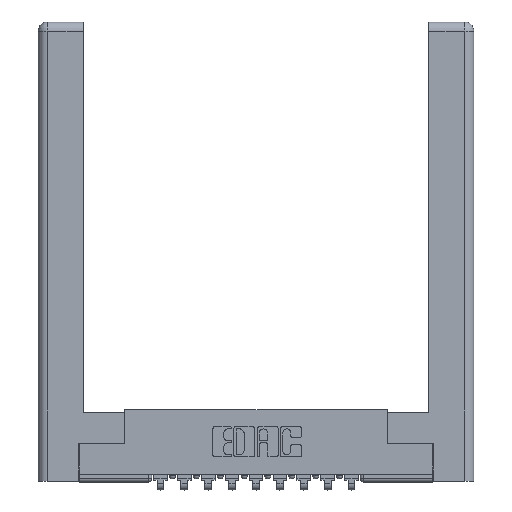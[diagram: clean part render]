
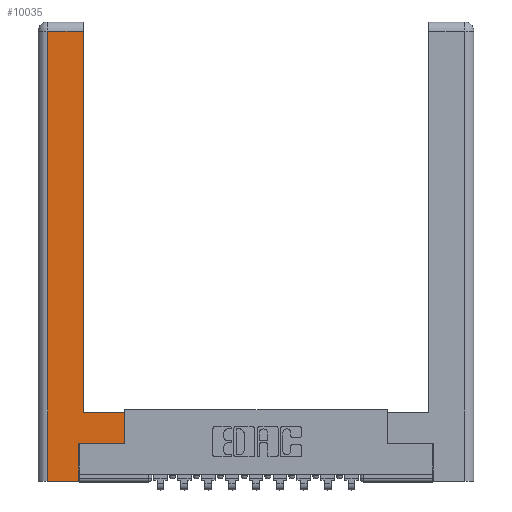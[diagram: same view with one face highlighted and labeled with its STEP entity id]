
A CAD part, top view. The second image highlights one B-rep face of the part: STEP entity #10035.
In plain terms, the highlighted planar face has unit normal (0, 0, 1).
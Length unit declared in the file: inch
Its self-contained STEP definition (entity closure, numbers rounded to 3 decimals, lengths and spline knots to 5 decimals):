
#168 = DIRECTION ( 'NONE',  ( 0., -1., 0. ) ) ;
#281 = CARTESIAN_POINT ( 'NONE',  ( 0., 0., 0. ) ) ;
#720 = ORIENTED_EDGE ( 'NONE', *, *, #9468, .T. ) ;
#917 = AXIS2_PLACEMENT_3D ( 'NONE', #281, #7357, #5945 ) ;
#1008 = LINE ( 'NONE', #1153, #5351 ) ;
#1153 = CARTESIAN_POINT ( 'NONE',  ( 0.265, 0., 0. ) ) ;
#1521 = EDGE_CURVE ( 'NONE', #10462, #13008, #4277, .T. ) ;
#1778 = CARTESIAN_POINT ( 'NONE',  ( 0.0615, 2.94, 0. ) ) ;
#1956 = VECTOR ( 'NONE', #4192, 39.37008 ) ;
#1999 = CARTESIAN_POINT ( 'NONE',  ( 0.565, 0.245, 0. ) ) ;
#2003 = FACE_OUTER_BOUND ( 'NONE', #11469, .T. ) ;
#2442 = EDGE_CURVE ( 'NONE', #12706, #10462, #7905, .T. ) ;
#2484 = LINE ( 'NONE', #15173, #7563 ) ;
#2895 = VERTEX_POINT ( 'NONE', #4299 ) ;
#2990 = DIRECTION ( 'NONE',  ( 0., 1., 0. ) ) ;
#4166 = EDGE_CURVE ( 'NONE', #12667, #4741, #8898, .T. ) ;
#4192 = DIRECTION ( 'NONE',  ( 0., 1., 0. ) ) ;
#4277 = LINE ( 'NONE', #9017, #11443 ) ;
#4299 = CARTESIAN_POINT ( 'NONE',  ( 0.0615, 0., 0. ) ) ;
#4522 = DIRECTION ( 'NONE',  ( -1., 0., 0. ) ) ;
#4537 = CARTESIAN_POINT ( 'NONE',  ( 0.565, 0.45, 0. ) ) ;
#4586 = DIRECTION ( 'NONE',  ( 0., 1., 0. ) ) ;
#4741 = VERTEX_POINT ( 'NONE', #5533 ) ;
#4830 = EDGE_CURVE ( 'NONE', #8221, #2895, #2484, .T. ) ;
#5008 = PLANE ( 'NONE',  #917 ) ;
#5012 = ORIENTED_EDGE ( 'NONE', *, *, #4166, .T. ) ;
#5351 = VECTOR ( 'NONE', #6982, 39.37008 ) ;
#5368 = ORIENTED_EDGE ( 'NONE', *, *, #1521, .T. ) ;
#5533 = CARTESIAN_POINT ( 'NONE',  ( 0.295, 2.94, 0. ) ) ;
#5945 = DIRECTION ( 'NONE',  ( -1., 0., 0. ) ) ;
#6275 = CARTESIAN_POINT ( 'NONE',  ( 0.0615, 2.94, 0. ) ) ;
#6533 = VECTOR ( 'NONE', #2990, 39.37008 ) ;
#6865 = LINE ( 'NONE', #9181, #9018 ) ;
#6982 = DIRECTION ( 'NONE',  ( 1., 0., 0. ) ) ;
#7357 = DIRECTION ( 'NONE',  ( 0., 0., -1. ) ) ;
#7432 = EDGE_CURVE ( 'NONE', #13008, #12667, #6865, .T. ) ;
#7563 = VECTOR ( 'NONE', #168, 39.37008 ) ;
#7771 = LINE ( 'NONE', #9230, #1956 ) ;
#7905 = LINE ( 'NONE', #1999, #8009 ) ;
#8009 = VECTOR ( 'NONE', #11531, 39.37008 ) ;
#8221 = VERTEX_POINT ( 'NONE', #1778 ) ;
#8533 = DIRECTION ( 'NONE',  ( -1., 0., 0. ) ) ;
#8642 = VECTOR ( 'NONE', #8533, 39.37008 ) ;
#8849 = VERTEX_POINT ( 'NONE', #13902 ) ;
#8898 = LINE ( 'NONE', #13583, #6533 ) ;
#9017 = CARTESIAN_POINT ( 'NONE',  ( 0.565, 0.45, 0. ) ) ;
#9018 = VECTOR ( 'NONE', #4522, 39.37008 ) ;
#9181 = CARTESIAN_POINT ( 'NONE',  ( 0.295, 0.45, 0. ) ) ;
#9230 = CARTESIAN_POINT ( 'NONE',  ( 0.265, 0.245, 0. ) ) ;
#9468 = EDGE_CURVE ( 'NONE', #2895, #8849, #1008, .T. ) ;
#9531 = LINE ( 'NONE', #6275, #8642 ) ;
#10032 = ORIENTED_EDGE ( 'NONE', *, *, #12495, .T. ) ;
#10035 = ADVANCED_FACE ( 'NONE', ( #2003 ), #5008, .F. ) ;
#10462 = VERTEX_POINT ( 'NONE', #12879 ) ;
#10886 = ORIENTED_EDGE ( 'NONE', *, *, #4830, .T. ) ;
#11110 = ORIENTED_EDGE ( 'NONE', *, *, #13773, .T. ) ;
#11443 = VECTOR ( 'NONE', #4586, 39.37008 ) ;
#11469 = EDGE_LOOP ( 'NONE', ( #5012, #11110, #10886, #720, #10032, #12124, #5368, #15278 ) ) ;
#11531 = DIRECTION ( 'NONE',  ( 1., 0., 0. ) ) ;
#12124 = ORIENTED_EDGE ( 'NONE', *, *, #2442, .T. ) ;
#12495 = EDGE_CURVE ( 'NONE', #8849, #12706, #7771, .T. ) ;
#12667 = VERTEX_POINT ( 'NONE', #13071 ) ;
#12706 = VERTEX_POINT ( 'NONE', #12850 ) ;
#12850 = CARTESIAN_POINT ( 'NONE',  ( 0.265, 0.245, 0. ) ) ;
#12879 = CARTESIAN_POINT ( 'NONE',  ( 0.565, 0.245, 0. ) ) ;
#13008 = VERTEX_POINT ( 'NONE', #4537 ) ;
#13071 = CARTESIAN_POINT ( 'NONE',  ( 0.295, 0.45, 0. ) ) ;
#13583 = CARTESIAN_POINT ( 'NONE',  ( 0.295, 3., 0. ) ) ;
#13773 = EDGE_CURVE ( 'NONE', #4741, #8221, #9531, .T. ) ;
#13902 = CARTESIAN_POINT ( 'NONE',  ( 0.265, 0., 0. ) ) ;
#15173 = CARTESIAN_POINT ( 'NONE',  ( 0.0615, 0., 0. ) ) ;
#15278 = ORIENTED_EDGE ( 'NONE', *, *, #7432, .T. ) ;
